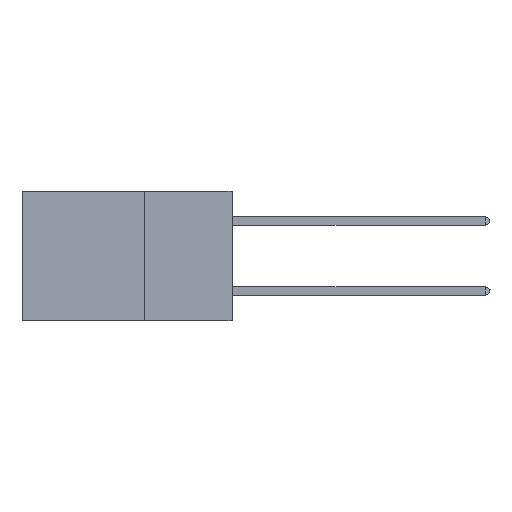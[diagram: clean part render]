
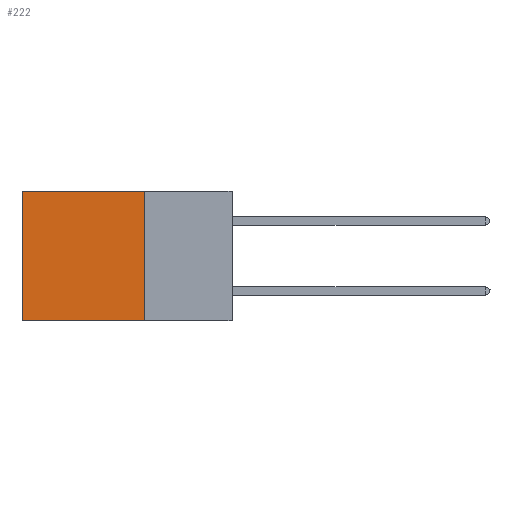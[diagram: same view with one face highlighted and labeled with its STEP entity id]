
A CAD part, left-side view. The second image highlights one B-rep face of the part: STEP entity #222.
In plain terms, the highlighted planar face has unit normal (-1, 0, 0).
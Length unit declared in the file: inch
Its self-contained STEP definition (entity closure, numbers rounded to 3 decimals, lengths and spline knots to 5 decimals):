
#222 = ADVANCED_FACE ( 'NONE', ( #3908 ), #1319, .F. ) ;
#922 = VERTEX_POINT ( 'NONE', #2432 ) ;
#1319 = PLANE ( 'NONE',  #2890 ) ;
#2432 = CARTESIAN_POINT ( 'NONE',  ( 0.2875, 0.6, -0.37 ) ) ;
#2879 = CARTESIAN_POINT ( 'NONE',  ( 0.2875, 0.25, 0. ) ) ;
#2890 = AXIS2_PLACEMENT_3D ( 'NONE', #2879, #13777, #8062 ) ;
#3101 = CARTESIAN_POINT ( 'NONE',  ( 0.2875, 0.25, 0. ) ) ;
#3788 = LINE ( 'NONE', #8768, #11455 ) ;
#3907 = CARTESIAN_POINT ( 'NONE',  ( 0.2875, 0.25, 0. ) ) ;
#3908 = FACE_OUTER_BOUND ( 'NONE', #16547, .T. ) ;
#4899 = CARTESIAN_POINT ( 'NONE',  ( 0.2875, 0.6, 0. ) ) ;
#5594 = ORIENTED_EDGE ( 'NONE', *, *, #16805, .T. ) ;
#5626 = ORIENTED_EDGE ( 'NONE', *, *, #11199, .F. ) ;
#5856 = DIRECTION ( 'NONE',  ( 0., 1., 0. ) ) ;
#6079 = VECTOR ( 'NONE', #8506, 39.37008 ) ;
#6710 = VECTOR ( 'NONE', #9308, 39.37008 ) ;
#7190 = VERTEX_POINT ( 'NONE', #9137 ) ;
#7547 = ORIENTED_EDGE ( 'NONE', *, *, #11244, .T. ) ;
#8024 = LINE ( 'NONE', #14997, #8665 ) ;
#8062 = DIRECTION ( 'NONE',  ( 0., 0., -1. ) ) ;
#8506 = DIRECTION ( 'NONE',  ( 0., 1., 0. ) ) ;
#8665 = VECTOR ( 'NONE', #12604, 39.37008 ) ;
#8768 = CARTESIAN_POINT ( 'NONE',  ( 0.2875, 0.25, -0.37 ) ) ;
#8799 = VERTEX_POINT ( 'NONE', #4899 ) ;
#9137 = CARTESIAN_POINT ( 'NONE',  ( 0.2875, 0.25, 0. ) ) ;
#9308 = DIRECTION ( 'NONE',  ( 0., 0., -1. ) ) ;
#9486 = LINE ( 'NONE', #3907, #6710 ) ;
#11183 = LINE ( 'NONE', #3101, #6079 ) ;
#11199 = EDGE_CURVE ( 'NONE', #14181, #922, #3788, .T. ) ;
#11244 = EDGE_CURVE ( 'NONE', #8799, #922, #8024, .T. ) ;
#11455 = VECTOR ( 'NONE', #5856, 39.37008 ) ;
#12209 = CARTESIAN_POINT ( 'NONE',  ( 0.2875, 0.25, -0.37 ) ) ;
#12604 = DIRECTION ( 'NONE',  ( 0., 0., -1. ) ) ;
#13777 = DIRECTION ( 'NONE',  ( 1., 0., 0. ) ) ;
#14181 = VERTEX_POINT ( 'NONE', #12209 ) ;
#14997 = CARTESIAN_POINT ( 'NONE',  ( 0.2875, 0.6, 0. ) ) ;
#15658 = ORIENTED_EDGE ( 'NONE', *, *, #16504, .F. ) ;
#16504 = EDGE_CURVE ( 'NONE', #7190, #14181, #9486, .T. ) ;
#16547 = EDGE_LOOP ( 'NONE', ( #7547, #5626, #15658, #5594 ) ) ;
#16805 = EDGE_CURVE ( 'NONE', #7190, #8799, #11183, .T. ) ;
